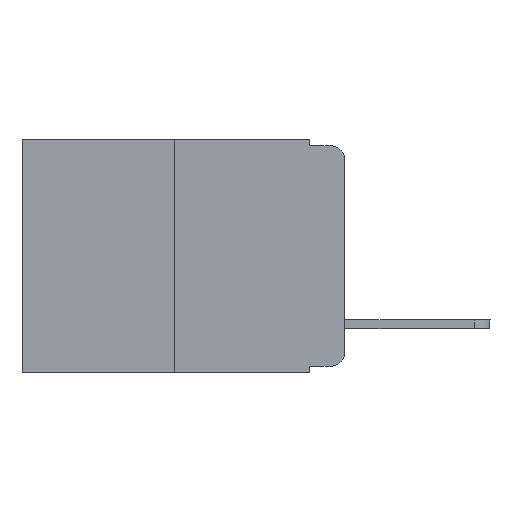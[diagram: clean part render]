
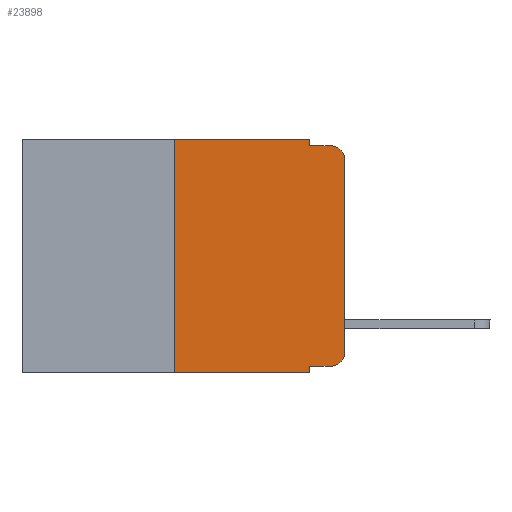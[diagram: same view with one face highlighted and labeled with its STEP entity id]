
A CAD part, left-side view. The second image highlights one B-rep face of the part: STEP entity #23898.
In plain terms, the highlighted planar face has unit normal (-1, 0, 0).
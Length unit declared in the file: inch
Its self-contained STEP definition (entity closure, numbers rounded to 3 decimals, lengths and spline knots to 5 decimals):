
#599 = LINE ( 'NONE', #15196, #18101 ) ;
#902 = LINE ( 'NONE', #12098, #5465 ) ;
#1204 = CARTESIAN_POINT ( 'NONE',  ( 0., 0., -0.313 ) ) ;
#1405 = DIRECTION ( 'NONE',  ( 0., 0., 1. ) ) ;
#1433 = DIRECTION ( 'NONE',  ( 0., 0., -1. ) ) ;
#1816 = EDGE_CURVE ( 'NONE', #3682, #4920, #15233, .T. ) ;
#1931 = DIRECTION ( 'NONE',  ( -1., 0., 0. ) ) ;
#2294 = EDGE_CURVE ( 'NONE', #2482, #15722, #2824, .T. ) ;
#2343 = VECTOR ( 'NONE', #1405, 39.37008 ) ;
#2365 = ORIENTED_EDGE ( 'NONE', *, *, #19090, .T. ) ;
#2482 = VERTEX_POINT ( 'NONE', #6833 ) ;
#2671 = LINE ( 'NONE', #19104, #5108 ) ;
#2694 = CARTESIAN_POINT ( 'NONE',  ( 0., 0.25, -0.343 ) ) ;
#2824 = CIRCLE ( 'NONE', #4616, 0.02 ) ;
#3282 = CARTESIAN_POINT ( 'NONE',  ( 0., 0.051, 0. ) ) ;
#3483 = VERTEX_POINT ( 'NONE', #22149 ) ;
#3632 = DIRECTION ( 'NONE',  ( 0., 0., 1. ) ) ;
#3682 = VERTEX_POINT ( 'NONE', #19843 ) ;
#3975 = LINE ( 'NONE', #14010, #13633 ) ;
#4452 = DIRECTION ( 'NONE',  ( 0., 0., -1. ) ) ;
#4616 = AXIS2_PLACEMENT_3D ( 'NONE', #14229, #18096, #4452 ) ;
#4696 = CARTESIAN_POINT ( 'NONE',  ( 0., 0.051, -0.01 ) ) ;
#4726 = DIRECTION ( 'NONE',  ( 1., 0., 0. ) ) ;
#4920 = VERTEX_POINT ( 'NONE', #4696 ) ;
#4937 = EDGE_CURVE ( 'NONE', #4920, #11782, #10147, .T. ) ;
#5047 = EDGE_CURVE ( 'NONE', #18572, #3682, #15871, .T. ) ;
#5108 = VECTOR ( 'NONE', #24879, 39.37008 ) ;
#5465 = VECTOR ( 'NONE', #6262, 39.37008 ) ;
#6203 = CARTESIAN_POINT ( 'NONE',  ( 0., 0.02, -0.01 ) ) ;
#6262 = DIRECTION ( 'NONE',  ( 0., -1., 0. ) ) ;
#6586 = PLANE ( 'NONE',  #7535 ) ;
#6833 = CARTESIAN_POINT ( 'NONE',  ( 0., 0.02, -0.333 ) ) ;
#7124 = CARTESIAN_POINT ( 'NONE',  ( 0., 0.473, 0. ) ) ;
#7535 = AXIS2_PLACEMENT_3D ( 'NONE', #23979, #4726, #12330 ) ;
#7720 = ORIENTED_EDGE ( 'NONE', *, *, #19473, .T. ) ;
#8445 = AXIS2_PLACEMENT_3D ( 'NONE', #13491, #1931, #15446 ) ;
#8483 = CARTESIAN_POINT ( 'NONE',  ( 0., 0.051, -0.01 ) ) ;
#9087 = DIRECTION ( 'NONE',  ( 0., -1., 0. ) ) ;
#9119 = FACE_OUTER_BOUND ( 'NONE', #9981, .T. ) ;
#9613 = ORIENTED_EDGE ( 'NONE', *, *, #4937, .F. ) ;
#9981 = EDGE_LOOP ( 'NONE', ( #7720, #15579, #9613, #16904, #23236, #10623, #14259, #21802, #2365, #20876 ) ) ;
#10147 = LINE ( 'NONE', #8483, #11975 ) ;
#10623 = ORIENTED_EDGE ( 'NONE', *, *, #21167, .F. ) ;
#11782 = VERTEX_POINT ( 'NONE', #6203 ) ;
#11975 = VECTOR ( 'NONE', #21922, 39.37008 ) ;
#12098 = CARTESIAN_POINT ( 'NONE',  ( 0., 0.051, -0.333 ) ) ;
#12330 = DIRECTION ( 'NONE',  ( 0., 0., -1. ) ) ;
#12614 = VERTEX_POINT ( 'NONE', #14512 ) ;
#12810 = VERTEX_POINT ( 'NONE', #2694 ) ;
#13491 = CARTESIAN_POINT ( 'NONE',  ( 0., 0.02, -0.03 ) ) ;
#13633 = VECTOR ( 'NONE', #21897, 39.37008 ) ;
#13819 = LINE ( 'NONE', #14561, #2343 ) ;
#14010 = CARTESIAN_POINT ( 'NONE',  ( 0., 0.051, 0. ) ) ;
#14229 = CARTESIAN_POINT ( 'NONE',  ( 0., 0.02, -0.313 ) ) ;
#14259 = ORIENTED_EDGE ( 'NONE', *, *, #17031, .T. ) ;
#14512 = CARTESIAN_POINT ( 'NONE',  ( 0., 0.051, -0.333 ) ) ;
#14561 = CARTESIAN_POINT ( 'NONE',  ( 0., 0.25, 0. ) ) ;
#15196 = CARTESIAN_POINT ( 'NONE',  ( 0., 0., 0. ) ) ;
#15233 = LINE ( 'NONE', #3282, #19141 ) ;
#15446 = DIRECTION ( 'NONE',  ( 0., 0., -1. ) ) ;
#15579 = ORIENTED_EDGE ( 'NONE', *, *, #19502, .T. ) ;
#15722 = VERTEX_POINT ( 'NONE', #1204 ) ;
#15871 = LINE ( 'NONE', #7124, #21554 ) ;
#16904 = ORIENTED_EDGE ( 'NONE', *, *, #1816, .F. ) ;
#17031 = EDGE_CURVE ( 'NONE', #12810, #3483, #2671, .T. ) ;
#18096 = DIRECTION ( 'NONE',  ( -1., 0., 0. ) ) ;
#18101 = VECTOR ( 'NONE', #3632, 39.37008 ) ;
#18411 = VERTEX_POINT ( 'NONE', #22151 ) ;
#18572 = VERTEX_POINT ( 'NONE', #22646 ) ;
#19090 = EDGE_CURVE ( 'NONE', #12614, #2482, #902, .T. ) ;
#19104 = CARTESIAN_POINT ( 'NONE',  ( 0., 0.473, -0.343 ) ) ;
#19141 = VECTOR ( 'NONE', #1433, 39.37008 ) ;
#19473 = EDGE_CURVE ( 'NONE', #15722, #18411, #599, .T. ) ;
#19502 = EDGE_CURVE ( 'NONE', #18411, #11782, #22585, .T. ) ;
#19843 = CARTESIAN_POINT ( 'NONE',  ( 0., 0.051, 0. ) ) ;
#20876 = ORIENTED_EDGE ( 'NONE', *, *, #2294, .T. ) ;
#21167 = EDGE_CURVE ( 'NONE', #12810, #18572, #13819, .T. ) ;
#21554 = VECTOR ( 'NONE', #9087, 39.37008 ) ;
#21802 = ORIENTED_EDGE ( 'NONE', *, *, #22853, .F. ) ;
#21897 = DIRECTION ( 'NONE',  ( 0., 0., -1. ) ) ;
#21922 = DIRECTION ( 'NONE',  ( 0., -1., 0. ) ) ;
#22149 = CARTESIAN_POINT ( 'NONE',  ( 0., 0.051, -0.343 ) ) ;
#22151 = CARTESIAN_POINT ( 'NONE',  ( 0., 0., -0.03 ) ) ;
#22585 = CIRCLE ( 'NONE', #8445, 0.02 ) ;
#22646 = CARTESIAN_POINT ( 'NONE',  ( 0., 0.25, 0. ) ) ;
#22853 = EDGE_CURVE ( 'NONE', #12614, #3483, #3975, .T. ) ;
#23236 = ORIENTED_EDGE ( 'NONE', *, *, #5047, .F. ) ;
#23898 = ADVANCED_FACE ( 'NONE', ( #9119 ), #6586, .F. ) ;
#23979 = CARTESIAN_POINT ( 'NONE',  ( 0., 0.473, 0. ) ) ;
#24879 = DIRECTION ( 'NONE',  ( 0., -1., 0. ) ) ;
